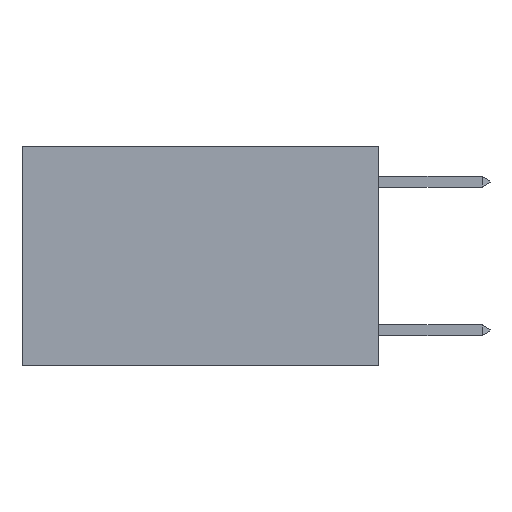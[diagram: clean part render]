
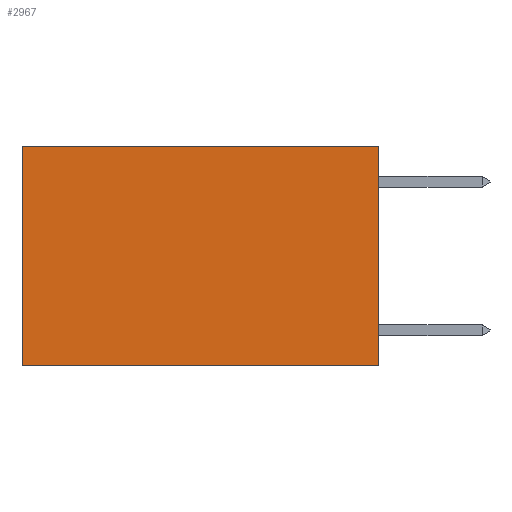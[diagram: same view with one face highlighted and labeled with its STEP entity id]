
A CAD part, left-side view. The second image highlights one B-rep face of the part: STEP entity #2967.
In plain terms, the highlighted planar face has unit normal (-1, 0, 0).
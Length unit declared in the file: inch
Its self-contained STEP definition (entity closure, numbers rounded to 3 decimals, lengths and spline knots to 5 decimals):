
#353 = LINE ( 'NONE', #14587, #10717 ) ;
#816 = DIRECTION ( 'NONE',  ( 1., 0., 0. ) ) ;
#978 = CARTESIAN_POINT ( 'NONE',  ( 0.2625, 0.6, 0. ) ) ;
#1597 = CARTESIAN_POINT ( 'NONE',  ( 0.2625, 0., 0. ) ) ;
#2354 = LINE ( 'NONE', #12797, #9384 ) ;
#2494 = EDGE_LOOP ( 'NONE', ( #5750, #14477, #8779, #14701 ) ) ;
#2520 = DIRECTION ( 'NONE',  ( 0., 1., 0. ) ) ;
#2772 = FACE_OUTER_BOUND ( 'NONE', #2494, .T. ) ;
#2842 = CARTESIAN_POINT ( 'NONE',  ( 0.2625, 0., -0.37 ) ) ;
#2967 = ADVANCED_FACE ( 'NONE', ( #2772 ), #12247, .F. ) ;
#3431 = VERTEX_POINT ( 'NONE', #5643 ) ;
#4202 = VERTEX_POINT ( 'NONE', #2842 ) ;
#4524 = VECTOR ( 'NONE', #5683, 39.37008 ) ;
#4558 = EDGE_CURVE ( 'NONE', #4202, #10090, #2354, .T. ) ;
#5643 = CARTESIAN_POINT ( 'NONE',  ( 0.2625, 0., 0. ) ) ;
#5683 = DIRECTION ( 'NONE',  ( 0., 0., -1. ) ) ;
#5750 = ORIENTED_EDGE ( 'NONE', *, *, #7886, .T. ) ;
#6814 = AXIS2_PLACEMENT_3D ( 'NONE', #1597, #816, #11388 ) ;
#6851 = LINE ( 'NONE', #978, #4524 ) ;
#7584 = EDGE_CURVE ( 'NONE', #3431, #4202, #353, .T. ) ;
#7690 = VECTOR ( 'NONE', #2520, 39.37008 ) ;
#7886 = EDGE_CURVE ( 'NONE', #8601, #10090, #6851, .T. ) ;
#8450 = CARTESIAN_POINT ( 'NONE',  ( 0.2625, 0.6, 0. ) ) ;
#8601 = VERTEX_POINT ( 'NONE', #8450 ) ;
#8779 = ORIENTED_EDGE ( 'NONE', *, *, #7584, .F. ) ;
#9210 = EDGE_CURVE ( 'NONE', #3431, #8601, #9565, .T. ) ;
#9384 = VECTOR ( 'NONE', #11868, 39.37008 ) ;
#9565 = LINE ( 'NONE', #13180, #7690 ) ;
#9811 = DIRECTION ( 'NONE',  ( 0., 0., -1. ) ) ;
#10090 = VERTEX_POINT ( 'NONE', #11740 ) ;
#10717 = VECTOR ( 'NONE', #9811, 39.37008 ) ;
#11388 = DIRECTION ( 'NONE',  ( 0., 0., -1. ) ) ;
#11740 = CARTESIAN_POINT ( 'NONE',  ( 0.2625, 0.6, -0.37 ) ) ;
#11868 = DIRECTION ( 'NONE',  ( 0., 1., 0. ) ) ;
#12247 = PLANE ( 'NONE',  #6814 ) ;
#12797 = CARTESIAN_POINT ( 'NONE',  ( 0.2625, 0., -0.37 ) ) ;
#13180 = CARTESIAN_POINT ( 'NONE',  ( 0.2625, 0., 0. ) ) ;
#14477 = ORIENTED_EDGE ( 'NONE', *, *, #4558, .F. ) ;
#14587 = CARTESIAN_POINT ( 'NONE',  ( 0.2625, 0., 0. ) ) ;
#14701 = ORIENTED_EDGE ( 'NONE', *, *, #9210, .T. ) ;
